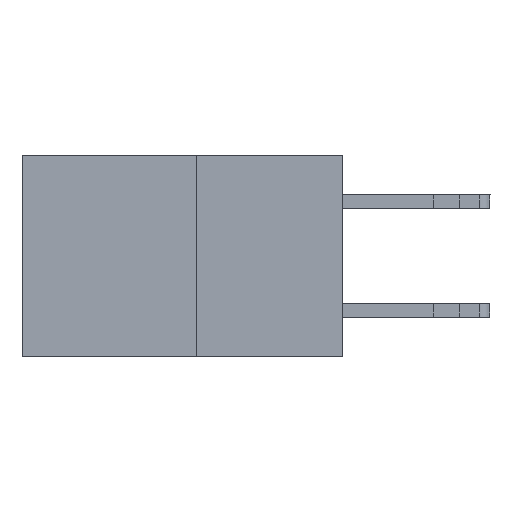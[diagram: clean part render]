
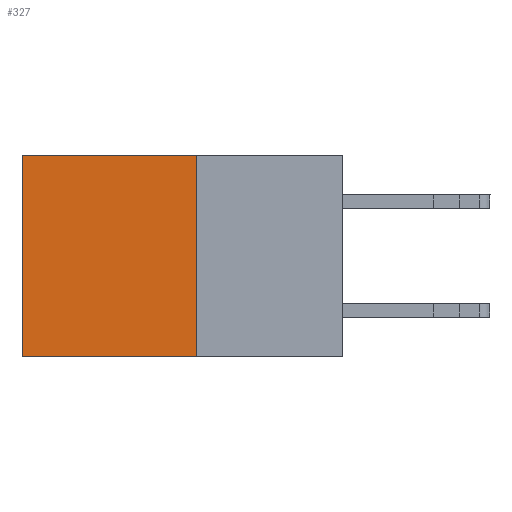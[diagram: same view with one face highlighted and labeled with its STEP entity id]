
A CAD part, left-side view. The second image highlights one B-rep face of the part: STEP entity #327.
In plain terms, the highlighted planar face has unit normal (-1, 0, 0).
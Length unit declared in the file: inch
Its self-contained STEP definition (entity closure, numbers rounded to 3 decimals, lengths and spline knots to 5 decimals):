
#287 = DIRECTION ( 'NONE',  ( 0., 1., 0. ) ) ;
#327 = ADVANCED_FACE ( 'NONE', ( #18965 ), #23809, .F. ) ;
#406 = VECTOR ( 'NONE', #1198, 39.37008 ) ;
#755 = LINE ( 'NONE', #16772, #12859 ) ;
#1198 = DIRECTION ( 'NONE',  ( 0., 0., -1. ) ) ;
#1849 = VERTEX_POINT ( 'NONE', #17799 ) ;
#2809 = LINE ( 'NONE', #12512, #32682 ) ;
#6090 = CARTESIAN_POINT ( 'NONE',  ( 0.277, 0.27, -0.37 ) ) ;
#6300 = DIRECTION ( 'NONE',  ( 0., 0., -1. ) ) ;
#6432 = DIRECTION ( 'NONE',  ( 1., 0., 0. ) ) ;
#6552 = CARTESIAN_POINT ( 'NONE',  ( 0.277, 0.59, -0.37 ) ) ;
#10350 = AXIS2_PLACEMENT_3D ( 'NONE', #6090, #6432, #26647 ) ;
#11077 = EDGE_LOOP ( 'NONE', ( #32225, #12818, #22422, #23854 ) ) ;
#12423 = CARTESIAN_POINT ( 'NONE',  ( 0.277, 0.59, 0. ) ) ;
#12512 = CARTESIAN_POINT ( 'NONE',  ( 0.277, 0.27, -0.37 ) ) ;
#12818 = ORIENTED_EDGE ( 'NONE', *, *, #18621, .F. ) ;
#12859 = VECTOR ( 'NONE', #15813, 39.37008 ) ;
#13897 = LINE ( 'NONE', #6552, #406 ) ;
#15605 = EDGE_CURVE ( 'NONE', #26575, #22896, #755, .T. ) ;
#15813 = DIRECTION ( 'NONE',  ( 0., 1., 0. ) ) ;
#16772 = CARTESIAN_POINT ( 'NONE',  ( 0.277, 0.27, 0. ) ) ;
#17799 = CARTESIAN_POINT ( 'NONE',  ( 0.277, 0.59, -0.37 ) ) ;
#18621 = EDGE_CURVE ( 'NONE', #29270, #1849, #2809, .T. ) ;
#18965 = FACE_OUTER_BOUND ( 'NONE', #11077, .T. ) ;
#21524 = CARTESIAN_POINT ( 'NONE',  ( 0.277, 0.27, -0.37 ) ) ;
#22422 = ORIENTED_EDGE ( 'NONE', *, *, #31160, .F. ) ;
#22896 = VERTEX_POINT ( 'NONE', #12423 ) ;
#23314 = EDGE_CURVE ( 'NONE', #22896, #1849, #13897, .T. ) ;
#23809 = PLANE ( 'NONE',  #10350 ) ;
#23854 = ORIENTED_EDGE ( 'NONE', *, *, #15605, .T. ) ;
#24193 = LINE ( 'NONE', #21524, #26330 ) ;
#26330 = VECTOR ( 'NONE', #6300, 39.37008 ) ;
#26575 = VERTEX_POINT ( 'NONE', #27565 ) ;
#26647 = DIRECTION ( 'NONE',  ( 0., 0., -1. ) ) ;
#27565 = CARTESIAN_POINT ( 'NONE',  ( 0.277, 0.27, 0. ) ) ;
#29270 = VERTEX_POINT ( 'NONE', #30763 ) ;
#30763 = CARTESIAN_POINT ( 'NONE',  ( 0.277, 0.27, -0.37 ) ) ;
#31160 = EDGE_CURVE ( 'NONE', #26575, #29270, #24193, .T. ) ;
#32225 = ORIENTED_EDGE ( 'NONE', *, *, #23314, .T. ) ;
#32682 = VECTOR ( 'NONE', #287, 39.37008 ) ;
